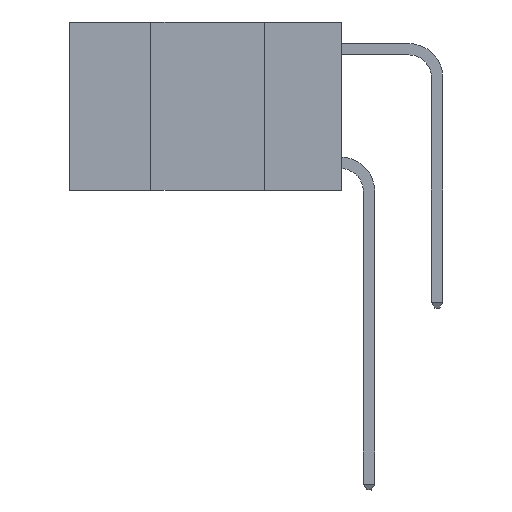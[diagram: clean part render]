
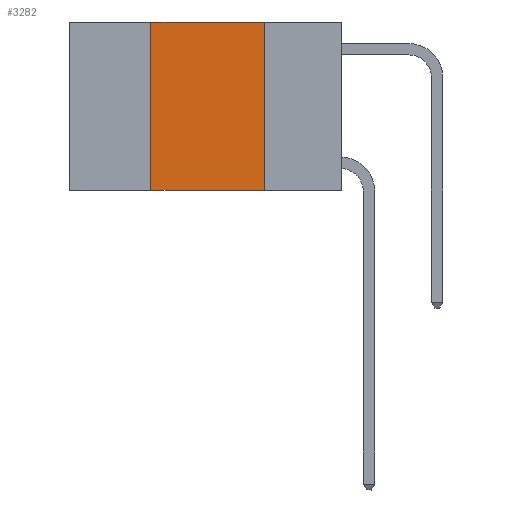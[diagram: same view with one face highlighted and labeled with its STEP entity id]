
A CAD part, left-side view. The second image highlights one B-rep face of the part: STEP entity #3282.
In plain terms, the highlighted planar face has unit normal (-1, 0, 0).
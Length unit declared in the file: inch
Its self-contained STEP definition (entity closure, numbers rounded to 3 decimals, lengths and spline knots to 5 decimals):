
#178 = CARTESIAN_POINT ( 'NONE',  ( 0., 0.42, 0. ) ) ;
#264 = ORIENTED_EDGE ( 'NONE', *, *, #18990, .F. ) ;
#362 = PLANE ( 'NONE',  #9482 ) ;
#415 = ORIENTED_EDGE ( 'NONE', *, *, #16882, .F. ) ;
#520 = DIRECTION ( 'NONE',  ( 1., 0., 0. ) ) ;
#1874 = ORIENTED_EDGE ( 'NONE', *, *, #23774, .F. ) ;
#3065 = CARTESIAN_POINT ( 'NONE',  ( 0., 0.17, 0. ) ) ;
#3214 = VERTEX_POINT ( 'NONE', #18942 ) ;
#3282 = ADVANCED_FACE ( 'NONE', ( #5570 ), #362, .F. ) ;
#3952 = CARTESIAN_POINT ( 'NONE',  ( 0., 0.6, 0. ) ) ;
#5024 = CARTESIAN_POINT ( 'NONE',  ( 0., 0.42, -0.37 ) ) ;
#5108 = VECTOR ( 'NONE', #9982, 39.37008 ) ;
#5570 = FACE_OUTER_BOUND ( 'NONE', #12640, .T. ) ;
#5671 = DIRECTION ( 'NONE',  ( 0., -1., 0. ) ) ;
#6633 = VECTOR ( 'NONE', #12407, 39.37008 ) ;
#7251 = DIRECTION ( 'NONE',  ( 0., 0., 1. ) ) ;
#7605 = CARTESIAN_POINT ( 'NONE',  ( 0., 0.6, -0.37 ) ) ;
#7809 = ORIENTED_EDGE ( 'NONE', *, *, #11046, .T. ) ;
#9482 = AXIS2_PLACEMENT_3D ( 'NONE', #3952, #520, #16853 ) ;
#9982 = DIRECTION ( 'NONE',  ( 0., 0., -1. ) ) ;
#10794 = CARTESIAN_POINT ( 'NONE',  ( 0., 0.42, 0. ) ) ;
#11046 = EDGE_CURVE ( 'NONE', #13340, #3214, #21343, .T. ) ;
#12407 = DIRECTION ( 'NONE',  ( 0., -1., 0. ) ) ;
#12640 = EDGE_LOOP ( 'NONE', ( #1874, #264, #415, #7809 ) ) ;
#13340 = VERTEX_POINT ( 'NONE', #5024 ) ;
#13561 = CARTESIAN_POINT ( 'NONE',  ( 0., 0.17, 0. ) ) ;
#14909 = VERTEX_POINT ( 'NONE', #3065 ) ;
#15628 = VERTEX_POINT ( 'NONE', #178 ) ;
#16853 = DIRECTION ( 'NONE',  ( 0., 0., -1. ) ) ;
#16882 = EDGE_CURVE ( 'NONE', #13340, #15628, #19166, .T. ) ;
#18942 = CARTESIAN_POINT ( 'NONE',  ( 0., 0.17, -0.37 ) ) ;
#18990 = EDGE_CURVE ( 'NONE', #15628, #14909, #21874, .T. ) ;
#19166 = LINE ( 'NONE', #10794, #22272 ) ;
#20074 = LINE ( 'NONE', #13561, #5108 ) ;
#21343 = LINE ( 'NONE', #7605, #23352 ) ;
#21551 = CARTESIAN_POINT ( 'NONE',  ( 0., 0.6, 0. ) ) ;
#21874 = LINE ( 'NONE', #21551, #6633 ) ;
#22272 = VECTOR ( 'NONE', #7251, 39.37008 ) ;
#23352 = VECTOR ( 'NONE', #5671, 39.37008 ) ;
#23774 = EDGE_CURVE ( 'NONE', #14909, #3214, #20074, .T. ) ;
